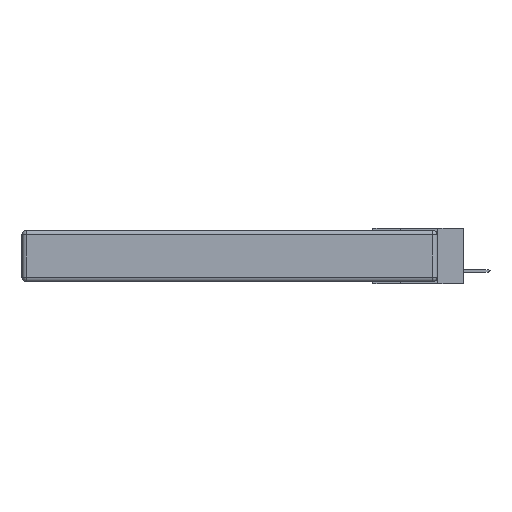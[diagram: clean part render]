
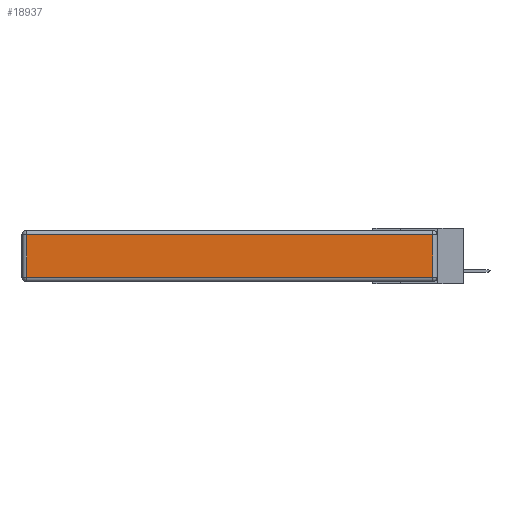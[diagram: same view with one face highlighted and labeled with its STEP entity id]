
A CAD part, left-side view. The second image highlights one B-rep face of the part: STEP entity #18937.
In plain terms, the highlighted planar face has unit normal (-1, 0, 0).
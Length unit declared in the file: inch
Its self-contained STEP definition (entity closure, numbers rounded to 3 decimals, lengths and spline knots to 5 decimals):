
#286 = EDGE_CURVE ( 'NONE', #7884, #989, #5309, .T. ) ;
#451 = CARTESIAN_POINT ( 'NONE',  ( 0., 2.72, -0.03 ) ) ;
#989 = VERTEX_POINT ( 'NONE', #10283 ) ;
#1028 = ORIENTED_EDGE ( 'NONE', *, *, #19758, .T. ) ;
#1148 = EDGE_CURVE ( 'NONE', #5604, #7884, #17722, .T. ) ;
#1711 = CARTESIAN_POINT ( 'NONE',  ( 0., 0., -0.343 ) ) ;
#2711 = CARTESIAN_POINT ( 'NONE',  ( 0., 0., -0.313 ) ) ;
#3113 = CARTESIAN_POINT ( 'NONE',  ( 0., 0.03, -0.03 ) ) ;
#3997 = DIRECTION ( 'NONE',  ( 0., 0., -1. ) ) ;
#4091 = DIRECTION ( 'NONE',  ( 0., -1., 0. ) ) ;
#5309 = LINE ( 'NONE', #2711, #15027 ) ;
#5496 = VECTOR ( 'NONE', #7741, 39.37008 ) ;
#5604 = VERTEX_POINT ( 'NONE', #451 ) ;
#5629 = VERTEX_POINT ( 'NONE', #3113 ) ;
#6018 = LINE ( 'NONE', #9222, #5496 ) ;
#6125 = ORIENTED_EDGE ( 'NONE', *, *, #286, .T. ) ;
#6753 = CARTESIAN_POINT ( 'NONE',  ( 0., 2.72, -0.313 ) ) ;
#7302 = CARTESIAN_POINT ( 'NONE',  ( 0., 2.72, -0.343 ) ) ;
#7717 = EDGE_LOOP ( 'NONE', ( #6125, #1028, #8000, #12964 ) ) ;
#7741 = DIRECTION ( 'NONE',  ( 0., 1., 0. ) ) ;
#7884 = VERTEX_POINT ( 'NONE', #6753 ) ;
#8000 = ORIENTED_EDGE ( 'NONE', *, *, #11119, .T. ) ;
#9222 = CARTESIAN_POINT ( 'NONE',  ( 0., 2.75, -0.03 ) ) ;
#9341 = PLANE ( 'NONE',  #12328 ) ;
#10283 = CARTESIAN_POINT ( 'NONE',  ( 0., 0.03, -0.313 ) ) ;
#11119 = EDGE_CURVE ( 'NONE', #5629, #5604, #6018, .T. ) ;
#11163 = LINE ( 'NONE', #16683, #19558 ) ;
#12328 = AXIS2_PLACEMENT_3D ( 'NONE', #1711, #12362, #18322 ) ;
#12362 = DIRECTION ( 'NONE',  ( -1., 0., 0. ) ) ;
#12696 = FACE_OUTER_BOUND ( 'NONE', #7717, .T. ) ;
#12964 = ORIENTED_EDGE ( 'NONE', *, *, #1148, .T. ) ;
#13265 = VECTOR ( 'NONE', #3997, 39.37008 ) ;
#15027 = VECTOR ( 'NONE', #4091, 39.37008 ) ;
#16683 = CARTESIAN_POINT ( 'NONE',  ( 0., 0.03, -0.343 ) ) ;
#17722 = LINE ( 'NONE', #7302, #13265 ) ;
#18223 = DIRECTION ( 'NONE',  ( 0., 0., 1. ) ) ;
#18322 = DIRECTION ( 'NONE',  ( 0., 0., 1. ) ) ;
#18937 = ADVANCED_FACE ( 'NONE', ( #12696 ), #9341, .T. ) ;
#19558 = VECTOR ( 'NONE', #18223, 39.37008 ) ;
#19758 = EDGE_CURVE ( 'NONE', #989, #5629, #11163, .T. ) ;
